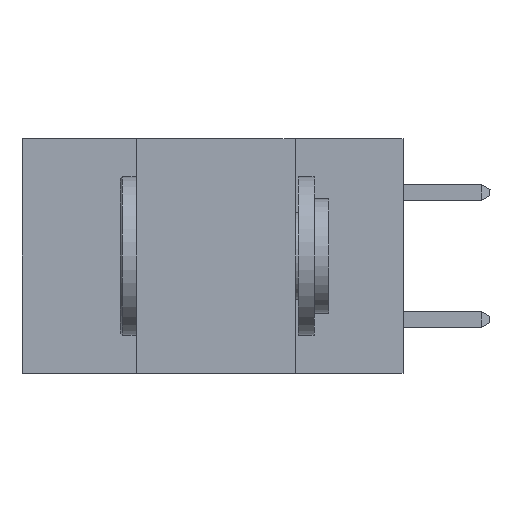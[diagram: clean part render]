
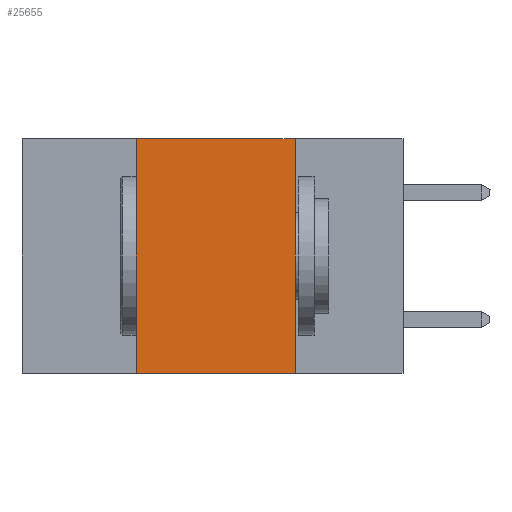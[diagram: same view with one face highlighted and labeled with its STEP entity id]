
A CAD part, left-side view. The second image highlights one B-rep face of the part: STEP entity #25655.
In plain terms, the highlighted planar face has unit normal (-1, 0, 0).
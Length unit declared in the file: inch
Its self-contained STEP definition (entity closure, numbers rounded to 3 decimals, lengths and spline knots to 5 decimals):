
#118 = DIRECTION ( 'NONE',  ( 0., 0., -1. ) ) ;
#586 = CARTESIAN_POINT ( 'NONE',  ( 0., 0.42, 0. ) ) ;
#647 = ORIENTED_EDGE ( 'NONE', *, *, #25412, .F. ) ;
#999 = CARTESIAN_POINT ( 'NONE',  ( 0., 0.42, 0. ) ) ;
#1268 = CARTESIAN_POINT ( 'NONE',  ( 0., 0.17, -0.37 ) ) ;
#1568 = VERTEX_POINT ( 'NONE', #999 ) ;
#2072 = LINE ( 'NONE', #4492, #10820 ) ;
#2631 = LINE ( 'NONE', #9842, #22103 ) ;
#2733 = VECTOR ( 'NONE', #6802, 39.37008 ) ;
#4492 = CARTESIAN_POINT ( 'NONE',  ( 0., 0.6, -0.37 ) ) ;
#4640 = CARTESIAN_POINT ( 'NONE',  ( 0., 0.17, 0. ) ) ;
#4876 = FACE_OUTER_BOUND ( 'NONE', #11091, .T. ) ;
#5430 = CARTESIAN_POINT ( 'NONE',  ( 0., 0.6, 0. ) ) ;
#5673 = EDGE_CURVE ( 'NONE', #1568, #23882, #11604, .T. ) ;
#6167 = CARTESIAN_POINT ( 'NONE',  ( 0., 0.6, 0. ) ) ;
#6802 = DIRECTION ( 'NONE',  ( 0., 0., 1. ) ) ;
#6977 = AXIS2_PLACEMENT_3D ( 'NONE', #6167, #14193, #118 ) ;
#9842 = CARTESIAN_POINT ( 'NONE',  ( 0., 0.17, 0. ) ) ;
#10820 = VECTOR ( 'NONE', #20580, 39.37008 ) ;
#11091 = EDGE_LOOP ( 'NONE', ( #17469, #17251, #647, #23462 ) ) ;
#11604 = LINE ( 'NONE', #5430, #22287 ) ;
#13548 = EDGE_CURVE ( 'NONE', #23060, #14198, #2072, .T. ) ;
#13784 = CARTESIAN_POINT ( 'NONE',  ( 0., 0.42, -0.37 ) ) ;
#14193 = DIRECTION ( 'NONE',  ( 1., 0., 0. ) ) ;
#14198 = VERTEX_POINT ( 'NONE', #1268 ) ;
#17251 = ORIENTED_EDGE ( 'NONE', *, *, #5673, .F. ) ;
#17469 = ORIENTED_EDGE ( 'NONE', *, *, #17696, .F. ) ;
#17696 = EDGE_CURVE ( 'NONE', #23882, #14198, #2631, .T. ) ;
#17829 = PLANE ( 'NONE',  #6977 ) ;
#19678 = LINE ( 'NONE', #586, #2733 ) ;
#20580 = DIRECTION ( 'NONE',  ( 0., -1., 0. ) ) ;
#22103 = VECTOR ( 'NONE', #25946, 39.37008 ) ;
#22287 = VECTOR ( 'NONE', #23622, 39.37008 ) ;
#23060 = VERTEX_POINT ( 'NONE', #13784 ) ;
#23462 = ORIENTED_EDGE ( 'NONE', *, *, #13548, .T. ) ;
#23622 = DIRECTION ( 'NONE',  ( 0., -1., 0. ) ) ;
#23882 = VERTEX_POINT ( 'NONE', #4640 ) ;
#25412 = EDGE_CURVE ( 'NONE', #23060, #1568, #19678, .T. ) ;
#25655 = ADVANCED_FACE ( 'NONE', ( #4876 ), #17829, .F. ) ;
#25946 = DIRECTION ( 'NONE',  ( 0., 0., -1. ) ) ;
